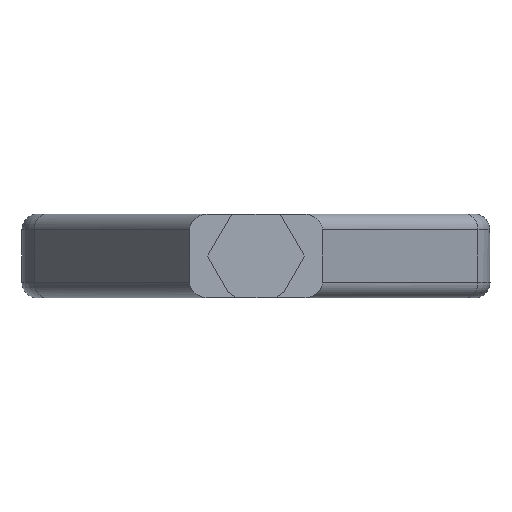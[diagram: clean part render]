
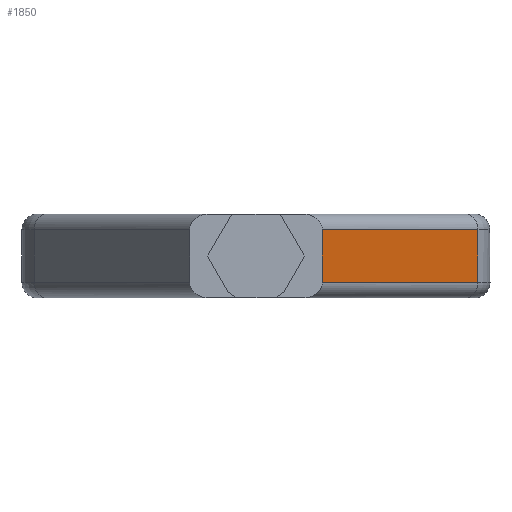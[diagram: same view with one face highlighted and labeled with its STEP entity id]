
A CAD part, front view. The second image highlights one B-rep face of the part: STEP entity #1850.
In plain terms, the highlighted planar face has unit normal (0.844, -0.536, 0).
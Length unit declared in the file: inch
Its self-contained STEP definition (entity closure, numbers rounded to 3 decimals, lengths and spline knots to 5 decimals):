
#8 = DIRECTION ( 'NONE',  ( -0.536, -0.844, 0. ) ) ;
#270 = CARTESIAN_POINT ( 'NONE',  ( 0.71108, 0.61604, -1.75948 ) ) ;
#284 = CARTESIAN_POINT ( 'NONE',  ( 0.21223, -0.17, -1.75948 ) ) ;
#512 = CARTESIAN_POINT ( 'NONE',  ( 0.21223, -0.17, 0.08455 ) ) ;
#550 = LINE ( 'NONE', #284, #1803 ) ;
#581 = CARTESIAN_POINT ( 'NONE',  ( 0.21223, -0.17, 0.08455 ) ) ;
#588 = ORIENTED_EDGE ( 'NONE', *, *, #984, .T. ) ;
#645 = VERTEX_POINT ( 'NONE', #581 ) ;
#692 = EDGE_LOOP ( 'NONE', ( #2005, #588, #1388, #1456 ) ) ;
#768 = VECTOR ( 'NONE', #1551, 39.37008 ) ;
#809 = DIRECTION ( 'NONE',  ( 0.844, -0.536, 0. ) ) ;
#814 = DIRECTION ( 'NONE',  ( 0., 0., 1. ) ) ;
#912 = VERTEX_POINT ( 'NONE', #1351 ) ;
#929 = VECTOR ( 'NONE', #814, 39.37008 ) ;
#961 = DIRECTION ( 'NONE',  ( 0., 0., 1. ) ) ;
#984 = EDGE_CURVE ( 'NONE', #1092, #2058, #1079, .T. ) ;
#987 = DIRECTION ( 'NONE',  ( 0.536, 0.844, 0. ) ) ;
#1079 = LINE ( 'NONE', #2095, #768 ) ;
#1092 = VERTEX_POINT ( 'NONE', #1219 ) ;
#1219 = CARTESIAN_POINT ( 'NONE',  ( 0.21223, -0.17, -0.08455 ) ) ;
#1264 = EDGE_CURVE ( 'NONE', #2058, #912, #1476, .T. ) ;
#1298 = EDGE_CURVE ( 'NONE', #1092, #645, #550, .T. ) ;
#1351 = CARTESIAN_POINT ( 'NONE',  ( 0.71108, 0.61604, 0.08455 ) ) ;
#1388 = ORIENTED_EDGE ( 'NONE', *, *, #1264, .T. ) ;
#1456 = ORIENTED_EDGE ( 'NONE', *, *, #1881, .T. ) ;
#1476 = LINE ( 'NONE', #270, #929 ) ;
#1551 = DIRECTION ( 'NONE',  ( 0.536, 0.844, 0. ) ) ;
#1569 = CARTESIAN_POINT ( 'NONE',  ( 0.71108, 0.61604, -0.08455 ) ) ;
#1746 = FACE_OUTER_BOUND ( 'NONE', #692, .T. ) ;
#1799 = LINE ( 'NONE', #512, #1853 ) ;
#1803 = VECTOR ( 'NONE', #961, 39.37008 ) ;
#1850 = ADVANCED_FACE ( 'NONE', ( #1746 ), #2183, .T. ) ;
#1853 = VECTOR ( 'NONE', #8, 39.37008 ) ;
#1881 = EDGE_CURVE ( 'NONE', #912, #645, #1799, .T. ) ;
#2005 = ORIENTED_EDGE ( 'NONE', *, *, #1298, .F. ) ;
#2058 = VERTEX_POINT ( 'NONE', #1569 ) ;
#2095 = CARTESIAN_POINT ( 'NONE',  ( 0.71108, 0.61604, -0.08455 ) ) ;
#2173 = AXIS2_PLACEMENT_3D ( 'NONE', #2220, #809, #987 ) ;
#2183 = PLANE ( 'NONE',  #2173 ) ;
#2220 = CARTESIAN_POINT ( 'NONE',  ( 0.21223, -0.17, -1.75948 ) ) ;
